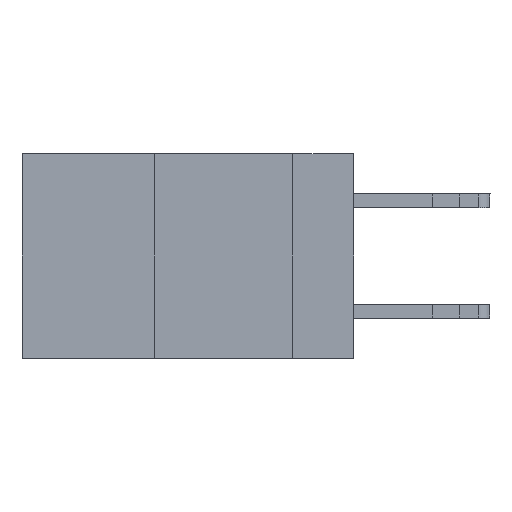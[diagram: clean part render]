
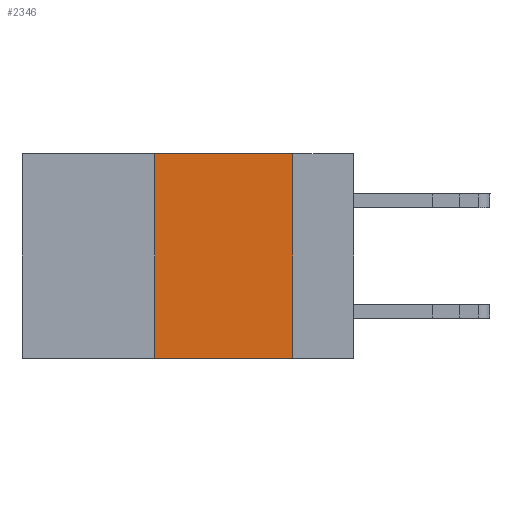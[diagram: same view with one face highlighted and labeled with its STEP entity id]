
A CAD part, left-side view. The second image highlights one B-rep face of the part: STEP entity #2346.
In plain terms, the highlighted planar face has unit normal (-1, 0, 0).
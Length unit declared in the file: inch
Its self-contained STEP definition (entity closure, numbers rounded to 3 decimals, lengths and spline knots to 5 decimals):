
#823 = VERTEX_POINT ( 'NONE', #7329 ) ;
#1402 = VERTEX_POINT ( 'NONE', #4297 ) ;
#1928 = VERTEX_POINT ( 'NONE', #2426 ) ;
#2250 = DIRECTION ( 'NONE',  ( 1., 0., 0. ) ) ;
#2346 = ADVANCED_FACE ( 'NONE', ( #2394 ), #11199, .F. ) ;
#2394 = FACE_OUTER_BOUND ( 'NONE', #3044, .T. ) ;
#2426 = CARTESIAN_POINT ( 'NONE',  ( 0., 0.36, -0.37 ) ) ;
#2451 = DIRECTION ( 'NONE',  ( 0., 0., 1. ) ) ;
#2539 = EDGE_CURVE ( 'NONE', #13640, #823, #21811, .T. ) ;
#3044 = EDGE_LOOP ( 'NONE', ( #13854, #4430, #14201, #16051 ) ) ;
#4248 = LINE ( 'NONE', #13753, #22288 ) ;
#4281 = EDGE_CURVE ( 'NONE', #823, #1402, #4248, .T. ) ;
#4297 = CARTESIAN_POINT ( 'NONE',  ( 0., 0.11, -0.37 ) ) ;
#4430 = ORIENTED_EDGE ( 'NONE', *, *, #2539, .F. ) ;
#5671 = VECTOR ( 'NONE', #16454, 39.37008 ) ;
#6673 = CARTESIAN_POINT ( 'NONE',  ( 0., 0.6, -0.37 ) ) ;
#7329 = CARTESIAN_POINT ( 'NONE',  ( 0., 0.11, 0. ) ) ;
#7882 = CARTESIAN_POINT ( 'NONE',  ( 0., 0.6, 0. ) ) ;
#8136 = EDGE_CURVE ( 'NONE', #1928, #1402, #9023, .T. ) ;
#9023 = LINE ( 'NONE', #6673, #14240 ) ;
#11199 = PLANE ( 'NONE',  #15218 ) ;
#12809 = CARTESIAN_POINT ( 'NONE',  ( 0., 0.6, 0. ) ) ;
#12939 = CARTESIAN_POINT ( 'NONE',  ( 0., 0.36, 0. ) ) ;
#13044 = DIRECTION ( 'NONE',  ( 0., 0., -1. ) ) ;
#13640 = VERTEX_POINT ( 'NONE', #20737 ) ;
#13753 = CARTESIAN_POINT ( 'NONE',  ( 0., 0.11, 0. ) ) ;
#13854 = ORIENTED_EDGE ( 'NONE', *, *, #4281, .F. ) ;
#14201 = ORIENTED_EDGE ( 'NONE', *, *, #20381, .F. ) ;
#14240 = VECTOR ( 'NONE', #18907, 39.37008 ) ;
#15218 = AXIS2_PLACEMENT_3D ( 'NONE', #12809, #2250, #13044 ) ;
#15676 = VECTOR ( 'NONE', #2451, 39.37008 ) ;
#16051 = ORIENTED_EDGE ( 'NONE', *, *, #8136, .T. ) ;
#16454 = DIRECTION ( 'NONE',  ( 0., -1., 0. ) ) ;
#17341 = DIRECTION ( 'NONE',  ( 0., 0., -1. ) ) ;
#18129 = LINE ( 'NONE', #12939, #15676 ) ;
#18907 = DIRECTION ( 'NONE',  ( 0., -1., 0. ) ) ;
#20381 = EDGE_CURVE ( 'NONE', #1928, #13640, #18129, .T. ) ;
#20737 = CARTESIAN_POINT ( 'NONE',  ( 0., 0.36, 0. ) ) ;
#21811 = LINE ( 'NONE', #7882, #5671 ) ;
#22288 = VECTOR ( 'NONE', #17341, 39.37008 ) ;
